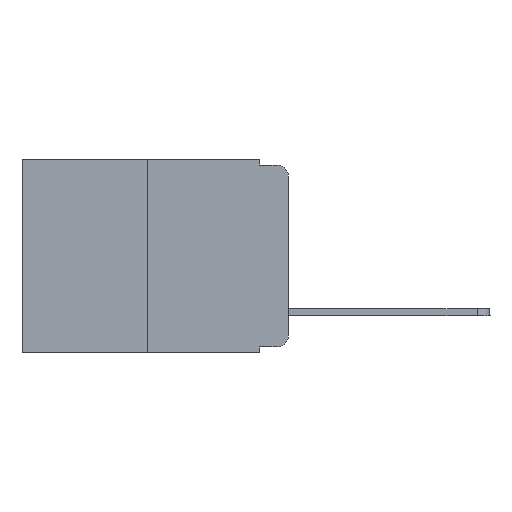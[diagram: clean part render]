
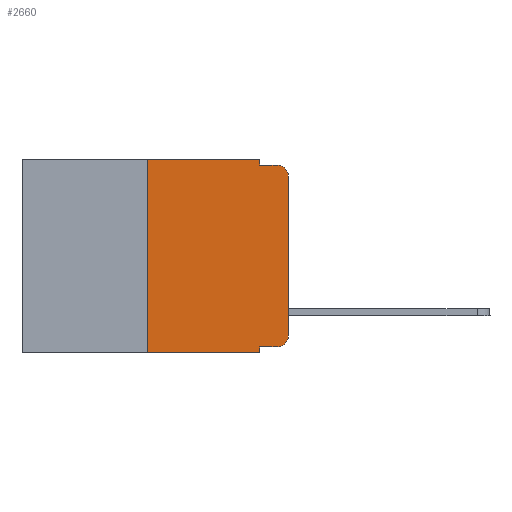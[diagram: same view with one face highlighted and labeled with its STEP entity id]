
A CAD part, left-side view. The second image highlights one B-rep face of the part: STEP entity #2660.
In plain terms, the highlighted planar face has unit normal (-1, 0, 0).
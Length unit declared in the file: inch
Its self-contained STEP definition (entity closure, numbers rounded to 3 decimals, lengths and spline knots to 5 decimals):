
#16 = VECTOR ( 'NONE', #2596, 39.37008 ) ;
#445 = VECTOR ( 'NONE', #7226, 39.37008 ) ;
#585 = AXIS2_PLACEMENT_3D ( 'NONE', #6219, #2422, #1378 ) ;
#1187 = EDGE_LOOP ( 'NONE', ( #4148, #11785, #8880, #4778, #1256, #9645, #5437, #7860, #6591, #5237 ) ) ;
#1188 = VERTEX_POINT ( 'NONE', #4157 ) ;
#1256 = ORIENTED_EDGE ( 'NONE', *, *, #3004, .F. ) ;
#1265 = VERTEX_POINT ( 'NONE', #7002 ) ;
#1338 = LINE ( 'NONE', #4615, #16 ) ;
#1378 = DIRECTION ( 'NONE',  ( 0., 0., -1. ) ) ;
#1507 = EDGE_CURVE ( 'NONE', #5302, #6031, #8616, .T. ) ;
#1648 = LINE ( 'NONE', #6296, #7405 ) ;
#1715 = DIRECTION ( 'NONE',  ( 0., -1., 0. ) ) ;
#2034 = CIRCLE ( 'NONE', #585, 0.02 ) ;
#2084 = VECTOR ( 'NONE', #9590, 39.37008 ) ;
#2090 = EDGE_CURVE ( 'NONE', #8931, #4350, #1648, .T. ) ;
#2201 = LINE ( 'NONE', #9309, #10615 ) ;
#2386 = VERTEX_POINT ( 'NONE', #9931 ) ;
#2422 = DIRECTION ( 'NONE',  ( -1., 0., 0. ) ) ;
#2497 = CARTESIAN_POINT ( 'NONE',  ( 0., 0.051, 0. ) ) ;
#2592 = DIRECTION ( 'NONE',  ( 0., -1., 0. ) ) ;
#2596 = DIRECTION ( 'NONE',  ( 0., 0., -1. ) ) ;
#2660 = ADVANCED_FACE ( 'NONE', ( #7554 ), #8478, .F. ) ;
#2815 = CARTESIAN_POINT ( 'NONE',  ( 0., 0.25, 0. ) ) ;
#2886 = EDGE_CURVE ( 'NONE', #5228, #4350, #1338, .T. ) ;
#3004 = EDGE_CURVE ( 'NONE', #1188, #9469, #3388, .T. ) ;
#3022 = EDGE_CURVE ( 'NONE', #10155, #2386, #2201, .T. ) ;
#3315 = EDGE_CURVE ( 'NONE', #8931, #1188, #11895, .T. ) ;
#3381 = VECTOR ( 'NONE', #5827, 39.37008 ) ;
#3388 = LINE ( 'NONE', #4625, #5319 ) ;
#3408 = DIRECTION ( 'NONE',  ( 0., -1., 0. ) ) ;
#3765 = CARTESIAN_POINT ( 'NONE',  ( 0., 0.051, -0.333 ) ) ;
#3792 = CIRCLE ( 'NONE', #6405, 0.02 ) ;
#3870 = EDGE_CURVE ( 'NONE', #2386, #6031, #2034, .T. ) ;
#4148 = ORIENTED_EDGE ( 'NONE', *, *, #3022, .T. ) ;
#4157 = CARTESIAN_POINT ( 'NONE',  ( 0., 0.25, 0. ) ) ;
#4350 = VERTEX_POINT ( 'NONE', #10037 ) ;
#4615 = CARTESIAN_POINT ( 'NONE',  ( 0., 0.051, 0. ) ) ;
#4625 = CARTESIAN_POINT ( 'NONE',  ( 0., 0.473, 0. ) ) ;
#4627 = CARTESIAN_POINT ( 'NONE',  ( 0., 0.02, -0.01 ) ) ;
#4754 = DIRECTION ( 'NONE',  ( -1., 0., 0. ) ) ;
#4778 = ORIENTED_EDGE ( 'NONE', *, *, #5435, .F. ) ;
#5228 = VERTEX_POINT ( 'NONE', #11509 ) ;
#5231 = VECTOR ( 'NONE', #2592, 39.37008 ) ;
#5237 = ORIENTED_EDGE ( 'NONE', *, *, #11893, .T. ) ;
#5302 = VERTEX_POINT ( 'NONE', #9898 ) ;
#5319 = VECTOR ( 'NONE', #1715, 39.37008 ) ;
#5435 = EDGE_CURVE ( 'NONE', #9469, #5302, #10753, .T. ) ;
#5437 = ORIENTED_EDGE ( 'NONE', *, *, #2090, .T. ) ;
#5467 = DIRECTION ( 'NONE',  ( 0., 0., 1. ) ) ;
#5827 = DIRECTION ( 'NONE',  ( 0., 0., 1. ) ) ;
#5921 = CARTESIAN_POINT ( 'NONE',  ( 0., 0.25, -0.343 ) ) ;
#6031 = VERTEX_POINT ( 'NONE', #4627 ) ;
#6219 = CARTESIAN_POINT ( 'NONE',  ( 0., 0.02, -0.03 ) ) ;
#6296 = CARTESIAN_POINT ( 'NONE',  ( 0., 0.473, -0.343 ) ) ;
#6405 = AXIS2_PLACEMENT_3D ( 'NONE', #7514, #4754, #6599 ) ;
#6591 = ORIENTED_EDGE ( 'NONE', *, *, #8266, .T. ) ;
#6599 = DIRECTION ( 'NONE',  ( 0., 0., -1. ) ) ;
#6837 = CARTESIAN_POINT ( 'NONE',  ( 0., 0.051, -0.01 ) ) ;
#7002 = CARTESIAN_POINT ( 'NONE',  ( 0., 0.02, -0.333 ) ) ;
#7226 = DIRECTION ( 'NONE',  ( 0., 0., -1. ) ) ;
#7405 = VECTOR ( 'NONE', #3408, 39.37008 ) ;
#7514 = CARTESIAN_POINT ( 'NONE',  ( 0., 0.02, -0.313 ) ) ;
#7554 = FACE_OUTER_BOUND ( 'NONE', #1187, .T. ) ;
#7820 = CARTESIAN_POINT ( 'NONE',  ( 0., 0.051, 0. ) ) ;
#7860 = ORIENTED_EDGE ( 'NONE', *, *, #2886, .F. ) ;
#7957 = AXIS2_PLACEMENT_3D ( 'NONE', #9559, #10346, #8604 ) ;
#8070 = LINE ( 'NONE', #3765, #5231 ) ;
#8266 = EDGE_CURVE ( 'NONE', #5228, #1265, #8070, .T. ) ;
#8478 = PLANE ( 'NONE',  #7957 ) ;
#8604 = DIRECTION ( 'NONE',  ( 0., 0., -1. ) ) ;
#8616 = LINE ( 'NONE', #6837, #2084 ) ;
#8880 = ORIENTED_EDGE ( 'NONE', *, *, #1507, .F. ) ;
#8931 = VERTEX_POINT ( 'NONE', #5921 ) ;
#9309 = CARTESIAN_POINT ( 'NONE',  ( 0., 0., 0. ) ) ;
#9469 = VERTEX_POINT ( 'NONE', #7820 ) ;
#9559 = CARTESIAN_POINT ( 'NONE',  ( 0., 0.473, 0. ) ) ;
#9590 = DIRECTION ( 'NONE',  ( 0., -1., 0. ) ) ;
#9645 = ORIENTED_EDGE ( 'NONE', *, *, #3315, .F. ) ;
#9898 = CARTESIAN_POINT ( 'NONE',  ( 0., 0.051, -0.01 ) ) ;
#9931 = CARTESIAN_POINT ( 'NONE',  ( 0., 0., -0.03 ) ) ;
#10037 = CARTESIAN_POINT ( 'NONE',  ( 0., 0.051, -0.343 ) ) ;
#10155 = VERTEX_POINT ( 'NONE', #11252 ) ;
#10346 = DIRECTION ( 'NONE',  ( 1., 0., 0. ) ) ;
#10615 = VECTOR ( 'NONE', #5467, 39.37008 ) ;
#10753 = LINE ( 'NONE', #2497, #445 ) ;
#11252 = CARTESIAN_POINT ( 'NONE',  ( 0., 0., -0.313 ) ) ;
#11509 = CARTESIAN_POINT ( 'NONE',  ( 0., 0.051, -0.333 ) ) ;
#11785 = ORIENTED_EDGE ( 'NONE', *, *, #3870, .T. ) ;
#11893 = EDGE_CURVE ( 'NONE', #1265, #10155, #3792, .T. ) ;
#11895 = LINE ( 'NONE', #2815, #3381 ) ;
